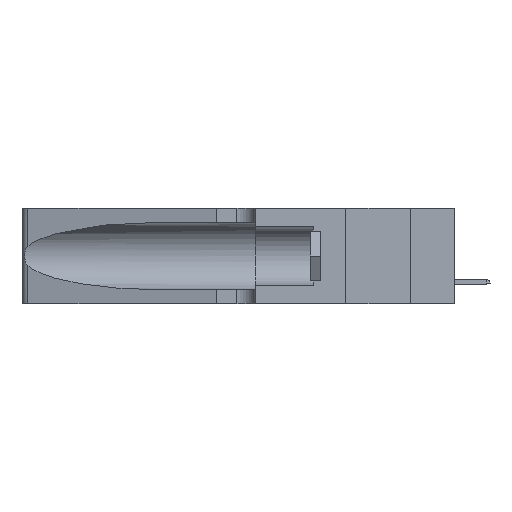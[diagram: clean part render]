
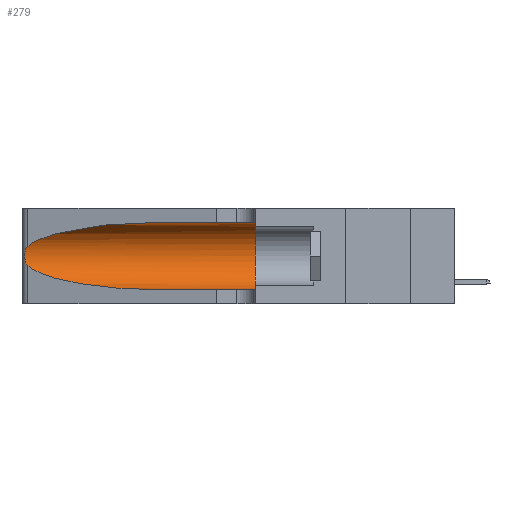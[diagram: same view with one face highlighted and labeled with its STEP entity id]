
A CAD part, left-side view. The second image highlights one B-rep face of the part: STEP entity #279.
In plain terms, the highlighted cylindrical face has radius 3.308 mm (diameter 6.617 mm), a partial arc.
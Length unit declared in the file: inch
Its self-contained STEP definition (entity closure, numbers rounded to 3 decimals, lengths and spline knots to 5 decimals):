
#171 = CARTESIAN_POINT ( 'NONE',  ( 0.25639, 1.23184, 0.21858 ) ) ;
#279 = ADVANCED_FACE ( 'NONE', ( #2380 ), #9630, .F. ) ;
#297 = CARTESIAN_POINT ( 'NONE',  ( 0.26075, 1.23896, 0.178 ) ) ;
#1026 = VERTEX_POINT ( 'NONE', #13446 ) ;
#1740 = AXIS2_PLACEMENT_3D ( 'NONE', #11761, #2720, #21002 ) ;
#1897 = CARTESIAN_POINT ( 'NONE',  ( 0.1305, 1.61858, 0.31525 ) ) ;
#2380 = FACE_OUTER_BOUND ( 'NONE', #19913, .T. ) ;
#2720 = DIRECTION ( 'NONE',  ( 0., 1., 0. ) ) ;
#3454 = CARTESIAN_POINT ( 'NONE',  ( 0.1305, 1.61858, 0.05475 ) ) ;
#3701 = CARTESIAN_POINT ( 'NONE',  ( 0.18966, 0.96281, 0.31525 ) ) ;
#4688 = CARTESIAN_POINT ( 'NONE',  ( 0.18966, 0.96281, 0.05475 ) ) ;
#5073 = DIRECTION ( 'NONE',  ( 0., 0., -1. ) ) ;
#5281 = ORIENTED_EDGE ( 'NONE', *, *, #18969, .F. ) ;
#5317 = DIRECTION ( 'NONE',  ( 0., -1., 0. ) ) ;
#5351 = ORIENTED_EDGE ( 'NONE', *, *, #16192, .F. ) ;
#5583 = CARTESIAN_POINT ( 'NONE',  ( 0.1305, 0.35, 0.31525 ) ) ;
#6295 = EDGE_CURVE ( 'NONE', #20028, #14183, #16855, .T. ) ;
#6591 = CARTESIAN_POINT ( 'NONE',  ( 0.1305, 0.72297, 0.05475 ) ) ;
#7019 = DIRECTION ( 'NONE',  ( 0., -1., 0. ) ) ;
#7322 = CARTESIAN_POINT ( 'NONE',  ( 0.25856, 1.23593, 0.16098 ) ) ;
#7563 = CARTESIAN_POINT ( 'NONE',  ( 0.25487, 1.22718, 0.14631 ) ) ;
#8260 = CARTESIAN_POINT ( 'NONE',  ( 0.2373, 1.15595, 0.08982 ) ) ;
#8306 = CARTESIAN_POINT ( 'NONE',  ( 0.1305, 0.72297, 0.05475 ) ) ;
#8694 = CARTESIAN_POINT ( 'NONE',  ( 0.2373, 1.15595, 0.28018 ) ) ;
#9216 = CARTESIAN_POINT ( 'NONE',  ( 0.25789, 1.23486, 0.15765 ) ) ;
#9260 = ORIENTED_EDGE ( 'NONE', *, *, #6295, .T. ) ;
#9357 =( BOUNDED_CURVE ( )  B_SPLINE_CURVE ( 3, ( #12477, #3701, #8694, #23400 ),
 .UNSPECIFIED., .F., .F. ) 
 B_SPLINE_CURVE_WITH_KNOTS ( ( 4, 4 ),
 ( 1.5708, 2.84003 ),
 .UNSPECIFIED. ) 
 CURVE ( )  GEOMETRIC_REPRESENTATION_ITEM ( )  RATIONAL_B_SPLINE_CURVE ( ( 1., 0.87, 0.87, 1. ) ) 
 REPRESENTATION_ITEM ( '' )  );
#9630 = CYLINDRICAL_SURFACE ( 'NONE', #21064, 0.13025 ) ;
#10909 = VECTOR ( 'NONE', #7019, 39.37008 ) ;
#11041 = CARTESIAN_POINT ( 'NONE',  ( 0.1305, 0.35, 0.05475 ) ) ;
#11116 = CARTESIAN_POINT ( 'NONE',  ( 0.25854, 1.2359, 0.20912 ) ) ;
#11446 = VERTEX_POINT ( 'NONE', #8306 ) ;
#11761 = CARTESIAN_POINT ( 'NONE',  ( 0.1305, 0.35, 0.185 ) ) ;
#12467 = DIRECTION ( 'NONE',  ( 0., -1., 0. ) ) ;
#12477 = CARTESIAN_POINT ( 'NONE',  ( 0.1305, 0.72297, 0.31525 ) ) ;
#12574 = LINE ( 'NONE', #3454, #10909 ) ;
#12650 = CARTESIAN_POINT ( 'NONE',  ( 0.25487, 1.22718, 0.22369 ) ) ;
#12665 =( BOUNDED_CURVE ( )  B_SPLINE_CURVE ( 3, ( #17471, #8260, #4688, #6591 ),
 .UNSPECIFIED., .F., .F. ) 
 B_SPLINE_CURVE_WITH_KNOTS ( ( 4, 4 ),
 ( 3.44316, 4.71239 ),
 .UNSPECIFIED. ) 
 CURVE ( )  GEOMETRIC_REPRESENTATION_ITEM ( )  RATIONAL_B_SPLINE_CURVE ( ( 1., 0.87, 0.87, 1. ) ) 
 REPRESENTATION_ITEM ( '' )  );
#13175 = VECTOR ( 'NONE', #12467, 39.37008 ) ;
#13446 = CARTESIAN_POINT ( 'NONE',  ( 0.1305, 0.72297, 0.31525 ) ) ;
#13647 = VERTEX_POINT ( 'NONE', #11041 ) ;
#14183 = VERTEX_POINT ( 'NONE', #16633 ) ;
#14548 = CARTESIAN_POINT ( 'NONE',  ( 0.26018, 1.23835, 0.19895 ) ) ;
#15236 = EDGE_CURVE ( 'NONE', #14183, #11446, #12665, .T. ) ;
#15561 = CARTESIAN_POINT ( 'NONE',  ( 0.25487, 1.22718, 0.22369 ) ) ;
#16192 = EDGE_CURVE ( 'NONE', #22609, #13647, #20726, .T. ) ;
#16358 = LINE ( 'NONE', #1897, #13175 ) ;
#16633 = CARTESIAN_POINT ( 'NONE',  ( 0.25487, 1.22718, 0.14631 ) ) ;
#16849 = CARTESIAN_POINT ( 'NONE',  ( 0.1305, 1.61858, 0.185 ) ) ;
#16855 = B_SPLINE_CURVE_WITH_KNOTS ( 'NONE', 3,
 ( #12650, #22147, #171, #21669, #11116, #14548, #17977, #297, #22029, #7322, #9216, #21794, #19892, #7563 ),
 .UNSPECIFIED., .F., .F.,
 ( 4, 2, 2, 2, 2, 2, 4 ),
 ( 0., 0.00027, 0.00053, 0.00107, 0.0016, 0.00187, 0.00214 ),
 .UNSPECIFIED. ) ;
#17124 = EDGE_CURVE ( 'NONE', #1026, #20028, #9357, .T. ) ;
#17471 = CARTESIAN_POINT ( 'NONE',  ( 0.25487, 1.22718, 0.14631 ) ) ;
#17977 = CARTESIAN_POINT ( 'NONE',  ( 0.26075, 1.23896, 0.19203 ) ) ;
#18969 = EDGE_CURVE ( 'NONE', #1026, #22609, #16358, .T. ) ;
#19001 = EDGE_CURVE ( 'NONE', #11446, #13647, #12574, .T. ) ;
#19892 = CARTESIAN_POINT ( 'NONE',  ( 0.25555, 1.22993, 0.14849 ) ) ;
#19913 = EDGE_LOOP ( 'NONE', ( #21878, #9260, #23221, #21488, #5351, #5281 ) ) ;
#20028 = VERTEX_POINT ( 'NONE', #15561 ) ;
#20726 = CIRCLE ( 'NONE', #1740, 0.13025 ) ;
#21002 = DIRECTION ( 'NONE',  ( 0., 0., 1. ) ) ;
#21064 = AXIS2_PLACEMENT_3D ( 'NONE', #16849, #5317, #5073 ) ;
#21488 = ORIENTED_EDGE ( 'NONE', *, *, #19001, .T. ) ;
#21669 = CARTESIAN_POINT ( 'NONE',  ( 0.25787, 1.23484, 0.2124 ) ) ;
#21794 = CARTESIAN_POINT ( 'NONE',  ( 0.25639, 1.23186, 0.15144 ) ) ;
#21878 = ORIENTED_EDGE ( 'NONE', *, *, #17124, .T. ) ;
#22029 = CARTESIAN_POINT ( 'NONE',  ( 0.26017, 1.23833, 0.17102 ) ) ;
#22147 = CARTESIAN_POINT ( 'NONE',  ( 0.25555, 1.22994, 0.2215 ) ) ;
#22609 = VERTEX_POINT ( 'NONE', #5583 ) ;
#23221 = ORIENTED_EDGE ( 'NONE', *, *, #15236, .T. ) ;
#23400 = CARTESIAN_POINT ( 'NONE',  ( 0.25487, 1.22718, 0.22369 ) ) ;
